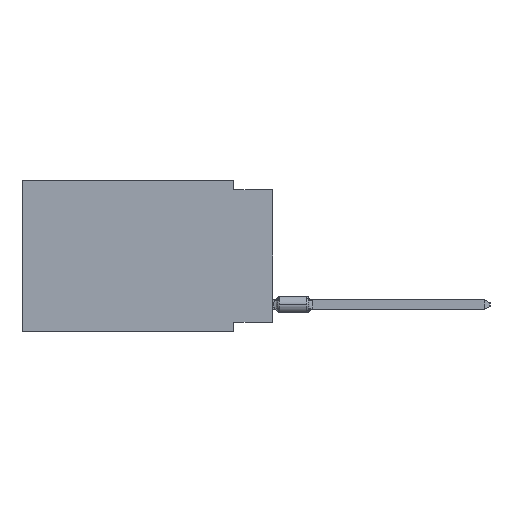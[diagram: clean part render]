
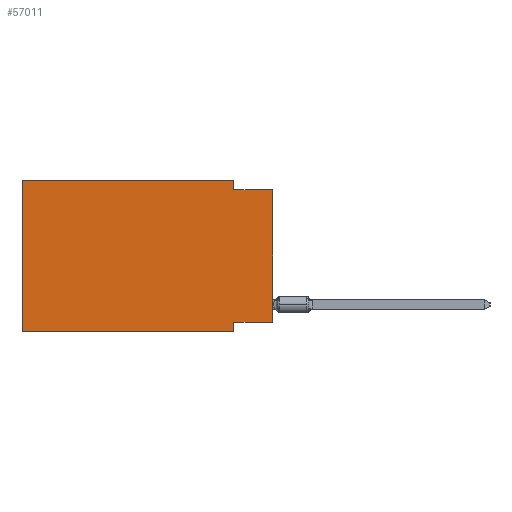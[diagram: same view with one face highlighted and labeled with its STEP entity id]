
A CAD part, left-side view. The second image highlights one B-rep face of the part: STEP entity #57011.
In plain terms, the highlighted planar face has unit normal (-1, 0, 0).
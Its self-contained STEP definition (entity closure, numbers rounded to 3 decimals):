
#1933 = ORIENTED_EDGE ( 'NONE', *, *, #11103, .F. ) ;
#2423 = CARTESIAN_POINT ( 'NONE',  ( 0., 0., -9.271 ) ) ;
#3484 = VECTOR ( 'NONE', #62167, 1000. ) ;
#4122 = ORIENTED_EDGE ( 'NONE', *, *, #59685, .F. ) ;
#4871 = VECTOR ( 'NONE', #22523, 1000. ) ;
#4973 = EDGE_CURVE ( 'NONE', #59120, #31097, #54550, .T. ) ;
#5306 = ORIENTED_EDGE ( 'NONE', *, *, #73450, .F. ) ;
#5326 = DIRECTION ( 'NONE',  ( 0., 0., 1. ) ) ;
#8198 = LINE ( 'NONE', #67157, #40732 ) ;
#9319 = LINE ( 'NONE', #69823, #35090 ) ;
#11103 = EDGE_CURVE ( 'NONE', #29118, #20253, #9319, .T. ) ;
#11317 = CARTESIAN_POINT ( 'NONE',  ( 0., 0., -0.635 ) ) ;
#12288 = CARTESIAN_POINT ( 'NONE',  ( 0., 16.383, 0. ) ) ;
#13712 = AXIS2_PLACEMENT_3D ( 'NONE', #46908, #65638, #41060 ) ;
#14101 = LINE ( 'NONE', #2423, #40887 ) ;
#14447 = VECTOR ( 'NONE', #5326, 1000. ) ;
#16027 = CARTESIAN_POINT ( 'NONE',  ( 0., 0., -9.271 ) ) ;
#17057 = VECTOR ( 'NONE', #49084, 1000. ) ;
#17087 = VERTEX_POINT ( 'NONE', #11317 ) ;
#17248 = FACE_OUTER_BOUND ( 'NONE', #59518, .T. ) ;
#20253 = VERTEX_POINT ( 'NONE', #39799 ) ;
#21040 = ORIENTED_EDGE ( 'NONE', *, *, #4973, .F. ) ;
#21514 = CARTESIAN_POINT ( 'NONE',  ( 0., 0., -0.635 ) ) ;
#22058 = CARTESIAN_POINT ( 'NONE',  ( 0., 2.54, -9.906 ) ) ;
#22523 = DIRECTION ( 'NONE',  ( 0., 0., -1. ) ) ;
#27603 = LINE ( 'NONE', #45575, #4871 ) ;
#28699 = CARTESIAN_POINT ( 'NONE',  ( 0., 0., 0. ) ) ;
#29118 = VERTEX_POINT ( 'NONE', #56169 ) ;
#31097 = VERTEX_POINT ( 'NONE', #40426 ) ;
#35090 = VECTOR ( 'NONE', #57306, 1000. ) ;
#36413 = EDGE_CURVE ( 'NONE', #65672, #47507, #27603, .T. ) ;
#36569 = CARTESIAN_POINT ( 'NONE',  ( 0., 16.383, -9.906 ) ) ;
#37965 = CARTESIAN_POINT ( 'NONE',  ( 0., 2.54, -9.271 ) ) ;
#39799 = CARTESIAN_POINT ( 'NONE',  ( 0., 2.54, -0.635 ) ) ;
#40426 = CARTESIAN_POINT ( 'NONE',  ( 0., 16.383, 0. ) ) ;
#40732 = VECTOR ( 'NONE', #60912, 1000. ) ;
#40887 = VECTOR ( 'NONE', #44153, 1000. ) ;
#41060 = DIRECTION ( 'NONE',  ( 0., 0., -1. ) ) ;
#41288 = EDGE_CURVE ( 'NONE', #20253, #17087, #75025, .T. ) ;
#41942 = DIRECTION ( 'NONE',  ( 0., -1., 0. ) ) ;
#43622 = CARTESIAN_POINT ( 'NONE',  ( 0., 16.383, 0. ) ) ;
#44153 = DIRECTION ( 'NONE',  ( 0., 1., 0. ) ) ;
#45575 = CARTESIAN_POINT ( 'NONE',  ( 0., 2.54, -9.906 ) ) ;
#46908 = CARTESIAN_POINT ( 'NONE',  ( 0., 16.383, 0. ) ) ;
#47507 = VERTEX_POINT ( 'NONE', #22058 ) ;
#49084 = DIRECTION ( 'NONE',  ( 0., 0., 1. ) ) ;
#50091 = ORIENTED_EDGE ( 'NONE', *, *, #76658, .T. ) ;
#53034 = ORIENTED_EDGE ( 'NONE', *, *, #54542, .T. ) ;
#53150 = PLANE ( 'NONE',  #13712 ) ;
#53652 = LINE ( 'NONE', #12288, #74882 ) ;
#54542 = EDGE_CURVE ( 'NONE', #61750, #17087, #58777, .T. ) ;
#54550 = LINE ( 'NONE', #43622, #17057 ) ;
#56169 = CARTESIAN_POINT ( 'NONE',  ( 0., 2.54, 0. ) ) ;
#56566 = ORIENTED_EDGE ( 'NONE', *, *, #36413, .F. ) ;
#57011 = ADVANCED_FACE ( 'NONE', ( #17248 ), #53150, .F. ) ;
#57306 = DIRECTION ( 'NONE',  ( 0., 0., -1. ) ) ;
#58777 = LINE ( 'NONE', #28699, #14447 ) ;
#59120 = VERTEX_POINT ( 'NONE', #36569 ) ;
#59518 = EDGE_LOOP ( 'NONE', ( #53034, #66857, #1933, #4122, #21040, #50091, #56566, #5306 ) ) ;
#59685 = EDGE_CURVE ( 'NONE', #31097, #29118, #53652, .T. ) ;
#60912 = DIRECTION ( 'NONE',  ( 0., -1., 0. ) ) ;
#61750 = VERTEX_POINT ( 'NONE', #16027 ) ;
#62167 = DIRECTION ( 'NONE',  ( 0., -1., 0. ) ) ;
#65638 = DIRECTION ( 'NONE',  ( 1., 0., 0. ) ) ;
#65672 = VERTEX_POINT ( 'NONE', #37965 ) ;
#66857 = ORIENTED_EDGE ( 'NONE', *, *, #41288, .F. ) ;
#67157 = CARTESIAN_POINT ( 'NONE',  ( 0., 16.383, -9.906 ) ) ;
#69823 = CARTESIAN_POINT ( 'NONE',  ( 0., 2.54, 0. ) ) ;
#73450 = EDGE_CURVE ( 'NONE', #61750, #65672, #14101, .T. ) ;
#74882 = VECTOR ( 'NONE', #41942, 1000. ) ;
#75025 = LINE ( 'NONE', #21514, #3484 ) ;
#76658 = EDGE_CURVE ( 'NONE', #59120, #47507, #8198, .T. ) ;
